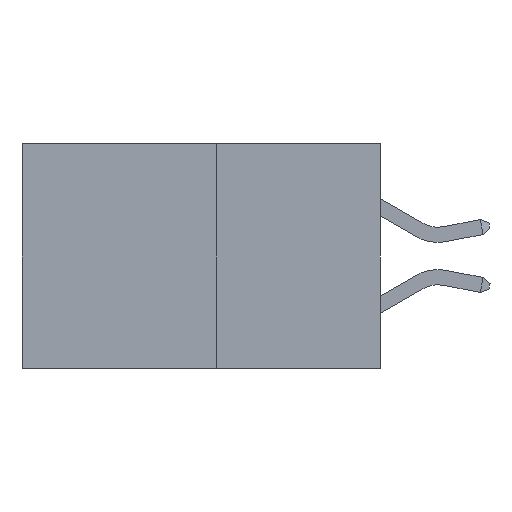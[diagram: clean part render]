
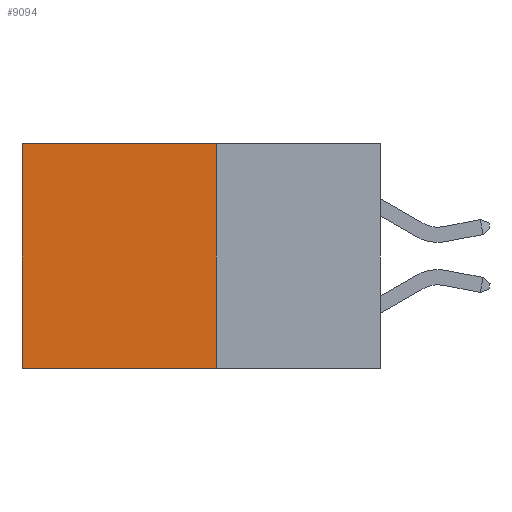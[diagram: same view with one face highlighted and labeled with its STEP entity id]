
A CAD part, left-side view. The second image highlights one B-rep face of the part: STEP entity #9094.
In plain terms, the highlighted planar face has unit normal (-1, 0, 0).
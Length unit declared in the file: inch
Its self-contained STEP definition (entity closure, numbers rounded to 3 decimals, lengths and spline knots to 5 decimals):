
#284 = VERTEX_POINT ( 'NONE', #13078 ) ;
#554 = DIRECTION ( 'NONE',  ( 0., 1., 0. ) ) ;
#1042 = DIRECTION ( 'NONE',  ( 0., 0., -1. ) ) ;
#1386 = LINE ( 'NONE', #1912, #6880 ) ;
#1648 = DIRECTION ( 'NONE',  ( 0., 0., -1. ) ) ;
#1912 = CARTESIAN_POINT ( 'NONE',  ( 0.277, 0.27, -0.37 ) ) ;
#2997 = EDGE_LOOP ( 'NONE', ( #9873, #10853, #4663, #15628 ) ) ;
#3425 = VERTEX_POINT ( 'NONE', #16964 ) ;
#3773 = VECTOR ( 'NONE', #554, 39.37008 ) ;
#4187 = EDGE_CURVE ( 'NONE', #12521, #3425, #1386, .T. ) ;
#4663 = ORIENTED_EDGE ( 'NONE', *, *, #4187, .F. ) ;
#5100 = CARTESIAN_POINT ( 'NONE',  ( 0.277, 0.59, -0.37 ) ) ;
#6415 = CARTESIAN_POINT ( 'NONE',  ( 0.277, 0.27, 0. ) ) ;
#6880 = VECTOR ( 'NONE', #1648, 39.37008 ) ;
#7779 = AXIS2_PLACEMENT_3D ( 'NONE', #14397, #24430, #12446 ) ;
#8583 = VECTOR ( 'NONE', #14906, 39.37008 ) ;
#8791 = CARTESIAN_POINT ( 'NONE',  ( 0.277, 0.27, -0.37 ) ) ;
#9094 = ADVANCED_FACE ( 'NONE', ( #19017 ), #20482, .F. ) ;
#9873 = ORIENTED_EDGE ( 'NONE', *, *, #19336, .T. ) ;
#10853 = ORIENTED_EDGE ( 'NONE', *, *, #14705, .F. ) ;
#12446 = DIRECTION ( 'NONE',  ( 0., 0., -1. ) ) ;
#12521 = VERTEX_POINT ( 'NONE', #6415 ) ;
#12860 = CARTESIAN_POINT ( 'NONE',  ( 0.277, 0.27, 0. ) ) ;
#13078 = CARTESIAN_POINT ( 'NONE',  ( 0.277, 0.59, 0. ) ) ;
#13955 = LINE ( 'NONE', #12860, #8583 ) ;
#14397 = CARTESIAN_POINT ( 'NONE',  ( 0.277, 0.27, -0.37 ) ) ;
#14705 = EDGE_CURVE ( 'NONE', #3425, #19767, #19953, .T. ) ;
#14721 = EDGE_CURVE ( 'NONE', #12521, #284, #13955, .T. ) ;
#14906 = DIRECTION ( 'NONE',  ( 0., 1., 0. ) ) ;
#15628 = ORIENTED_EDGE ( 'NONE', *, *, #14721, .T. ) ;
#16554 = CARTESIAN_POINT ( 'NONE',  ( 0.277, 0.59, -0.37 ) ) ;
#16964 = CARTESIAN_POINT ( 'NONE',  ( 0.277, 0.27, -0.37 ) ) ;
#19017 = FACE_OUTER_BOUND ( 'NONE', #2997, .T. ) ;
#19214 = LINE ( 'NONE', #5100, #23189 ) ;
#19336 = EDGE_CURVE ( 'NONE', #284, #19767, #19214, .T. ) ;
#19767 = VERTEX_POINT ( 'NONE', #16554 ) ;
#19953 = LINE ( 'NONE', #8791, #3773 ) ;
#20482 = PLANE ( 'NONE',  #7779 ) ;
#23189 = VECTOR ( 'NONE', #1042, 39.37008 ) ;
#24430 = DIRECTION ( 'NONE',  ( 1., 0., 0. ) ) ;
